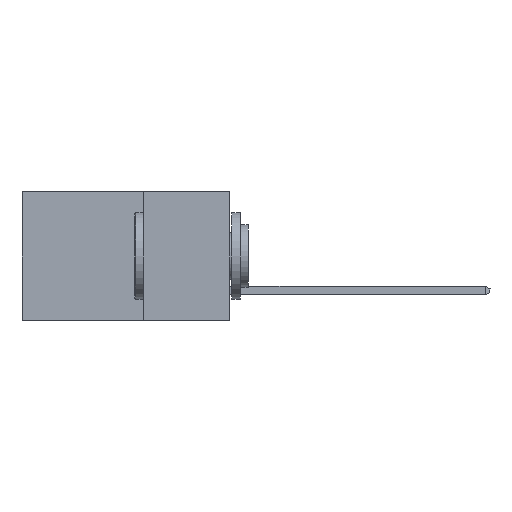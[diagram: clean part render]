
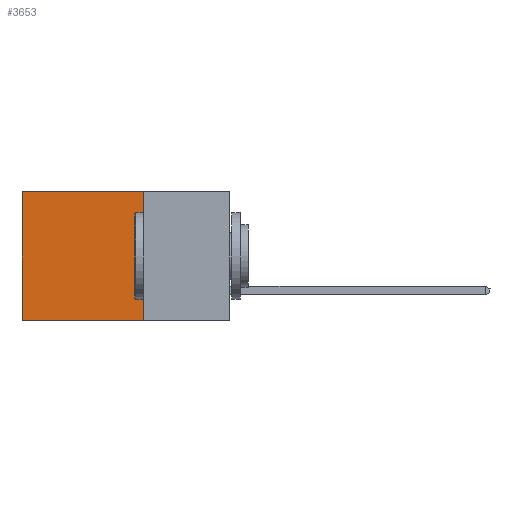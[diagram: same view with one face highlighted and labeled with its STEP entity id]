
A CAD part, left-side view. The second image highlights one B-rep face of the part: STEP entity #3653.
In plain terms, the highlighted planar face has unit normal (-1, 0, 0).
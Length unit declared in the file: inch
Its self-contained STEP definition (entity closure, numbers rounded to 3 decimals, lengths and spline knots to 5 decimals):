
#767 = ORIENTED_EDGE ( 'NONE', *, *, #3782, .T. ) ;
#984 = DIRECTION ( 'NONE',  ( 0., 1., 0. ) ) ;
#1334 = CARTESIAN_POINT ( 'NONE',  ( 0.2615, 0.25, -0.37 ) ) ;
#1767 = CARTESIAN_POINT ( 'NONE',  ( 0.2615, 0.6, 0. ) ) ;
#2497 = AXIS2_PLACEMENT_3D ( 'NONE', #9701, #7832, #16388 ) ;
#2931 = VECTOR ( 'NONE', #19685, 39.37008 ) ;
#3653 = ADVANCED_FACE ( 'NONE', ( #19952 ), #4047, .F. ) ;
#3782 = EDGE_CURVE ( 'NONE', #20775, #7964, #12492, .T. ) ;
#4047 = PLANE ( 'NONE',  #2497 ) ;
#4994 = DIRECTION ( 'NONE',  ( 0., 0., -1. ) ) ;
#5109 = ORIENTED_EDGE ( 'NONE', *, *, #21279, .F. ) ;
#5399 = DIRECTION ( 'NONE',  ( 0., 0., -1. ) ) ;
#5431 = EDGE_CURVE ( 'NONE', #19525, #13378, #15329, .T. ) ;
#6601 = ORIENTED_EDGE ( 'NONE', *, *, #5431, .F. ) ;
#7161 = CARTESIAN_POINT ( 'NONE',  ( 0.2615, 0.25, -0.37 ) ) ;
#7359 = VECTOR ( 'NONE', #4994, 39.37008 ) ;
#7832 = DIRECTION ( 'NONE',  ( 1., 0., 0. ) ) ;
#7964 = VERTEX_POINT ( 'NONE', #1767 ) ;
#8478 = ORIENTED_EDGE ( 'NONE', *, *, #9271, .T. ) ;
#8923 = LINE ( 'NONE', #7161, #18052 ) ;
#9177 = CARTESIAN_POINT ( 'NONE',  ( 0.2615, 0.25, 0. ) ) ;
#9271 = EDGE_CURVE ( 'NONE', #7964, #13378, #22773, .T. ) ;
#9701 = CARTESIAN_POINT ( 'NONE',  ( 0.2615, 0.25, -0.37 ) ) ;
#12492 = LINE ( 'NONE', #15341, #2931 ) ;
#13237 = VECTOR ( 'NONE', #984, 39.37008 ) ;
#13378 = VERTEX_POINT ( 'NONE', #20103 ) ;
#14032 = CARTESIAN_POINT ( 'NONE',  ( 0.2615, 0.6, -0.37 ) ) ;
#15329 = LINE ( 'NONE', #16975, #13237 ) ;
#15341 = CARTESIAN_POINT ( 'NONE',  ( 0.2615, 0.25, 0. ) ) ;
#16388 = DIRECTION ( 'NONE',  ( 0., 0., -1. ) ) ;
#16975 = CARTESIAN_POINT ( 'NONE',  ( 0.2615, 0.25, -0.37 ) ) ;
#18052 = VECTOR ( 'NONE', #5399, 39.37008 ) ;
#19525 = VERTEX_POINT ( 'NONE', #1334 ) ;
#19685 = DIRECTION ( 'NONE',  ( 0., 1., 0. ) ) ;
#19952 = FACE_OUTER_BOUND ( 'NONE', #20675, .T. ) ;
#20103 = CARTESIAN_POINT ( 'NONE',  ( 0.2615, 0.6, -0.37 ) ) ;
#20675 = EDGE_LOOP ( 'NONE', ( #8478, #6601, #5109, #767 ) ) ;
#20775 = VERTEX_POINT ( 'NONE', #9177 ) ;
#21279 = EDGE_CURVE ( 'NONE', #20775, #19525, #8923, .T. ) ;
#22773 = LINE ( 'NONE', #14032, #7359 ) ;
